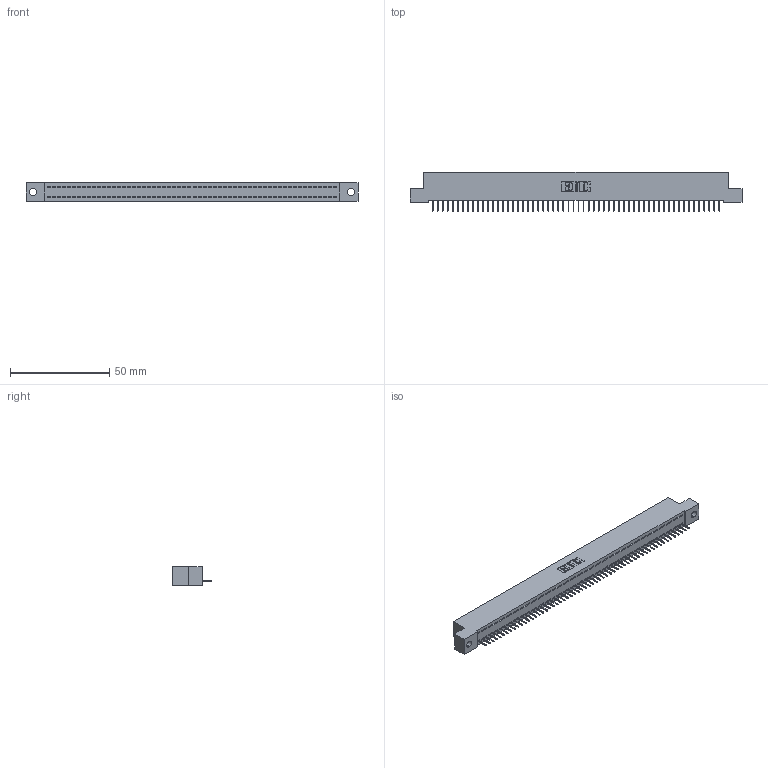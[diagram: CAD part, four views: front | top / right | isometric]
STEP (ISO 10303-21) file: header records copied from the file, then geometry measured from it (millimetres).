
FILE_DESCRIPTION (( 'STEP AP203' ), '1' );
FILE_NAME ('392-058-524-102.STEP', '2018-08-17T16:34:08', ( '' ), ( '' ), 'SwSTEP 2.0', 'SolidWorks 2016', '' );
FILE_SCHEMA (( 'CONFIG_CONTROL_DESIGN' ));
Length unit declared in the file: inch
Products named in the file (3): 342 Part_.128 Slot; 345-292-001_345-293-124; 392-058-524-102
Assembly tree (59 placements, depth 2):
  392-058-524-102
    342 Part_.128 Slot
    345-292-001_345-293-124  x58
Bounding box: 167.64 x 19.69 x 9.4 mm (x, y, z)
Volume: 14476.4 mm3; surface area: 20604.6 mm2
Topology: 59 solids, 59 shells, 3710 faces, 10751 edges, 6934 vertices
Faces by surface type: plane 2854, cylinder 856
Entity records: 33465 total; most frequent: CARTESIAN_POINT 5776, ORIENTED_EDGE 5770, DIRECTION 4841, EDGE_CURVE 2885, LINE 2761, VECTOR 2761, VERTEX_POINT 1918, AXIS2_PLACEMENT_3D 1040
